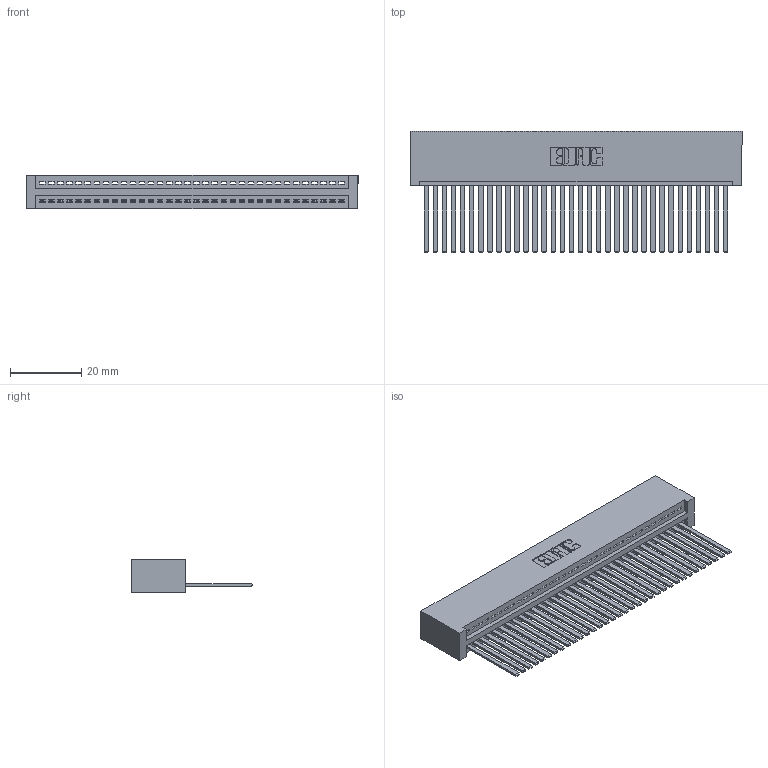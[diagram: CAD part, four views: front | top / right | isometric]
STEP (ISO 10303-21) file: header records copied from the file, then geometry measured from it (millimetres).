
FILE_DESCRIPTION (( 'STEP AP203' ), '1' );
FILE_NAME ('395-034-544-101.STEP', '2019-10-19T18:05:24', ( '' ), ( '' ), 'SwSTEP 2.0', 'SolidWorks 2016', '' );
FILE_SCHEMA (( 'CONFIG_CONTROL_DESIGN' ));
Length unit declared in the file: inch
Products named in the file (3): 345 Part_No Mounting Lugs; 345-292-001_345-293-144; 395-034-544-101
Assembly tree (35 placements, depth 2):
  395-034-544-101
    345 Part_No Mounting Lugs
    345-292-001_345-293-144  x34
Bounding box: 92.96 x 33.96 x 9.4 mm (x, y, z)
Volume: 9742.4 mm3; surface area: 14210.3 mm2
Topology: 35 solids, 35 shells, 1886 faces, 5689 edges, 3746 vertices
Faces by surface type: plane 1300, cylinder 586
Entity records: 26205 total; most frequent: CARTESIAN_POINT 4546, ORIENTED_EDGE 4514, DIRECTION 3973, EDGE_CURVE 2257, VECTOR 2001, LINE 2001, VERTEX_POINT 1502, AXIS2_PLACEMENT_3D 986
